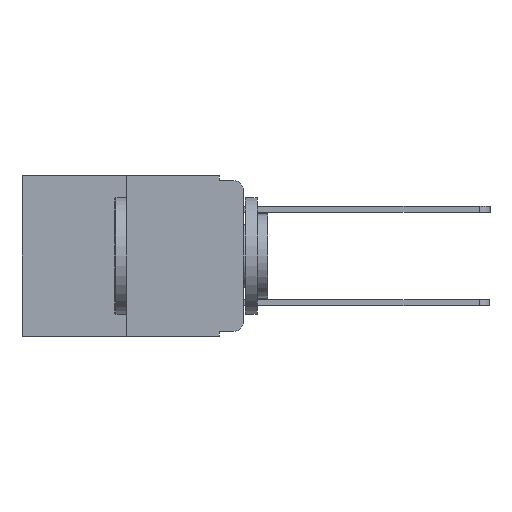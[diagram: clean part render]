
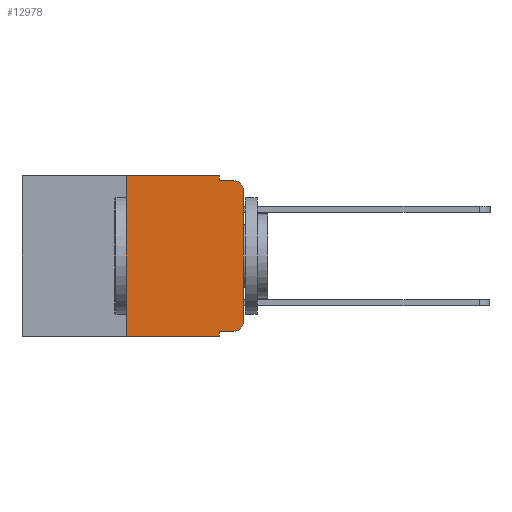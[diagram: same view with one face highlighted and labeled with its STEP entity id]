
A CAD part, left-side view. The second image highlights one B-rep face of the part: STEP entity #12978.
In plain terms, the highlighted planar face has unit normal (-1, 0, 0).
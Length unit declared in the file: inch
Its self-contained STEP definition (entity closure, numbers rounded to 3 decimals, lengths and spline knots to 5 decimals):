
#247 = DIRECTION ( 'NONE',  ( 0., 0., -1. ) ) ;
#1131 = DIRECTION ( 'NONE',  ( 0., 0., 1. ) ) ;
#1620 = CARTESIAN_POINT ( 'NONE',  ( 0., 0.051, 0. ) ) ;
#1825 = DIRECTION ( 'NONE',  ( -1., 0., 0. ) ) ;
#1891 = EDGE_CURVE ( 'NONE', #11463, #6679, #20076, .T. ) ;
#2016 = VERTEX_POINT ( 'NONE', #11448 ) ;
#2154 = ORIENTED_EDGE ( 'NONE', *, *, #18420, .F. ) ;
#2264 = AXIS2_PLACEMENT_3D ( 'NONE', #14364, #10949, #247 ) ;
#2492 = CARTESIAN_POINT ( 'NONE',  ( 0., 0.051, -0.01 ) ) ;
#2641 = CARTESIAN_POINT ( 'NONE',  ( 0., 0., -0.313 ) ) ;
#2963 = CARTESIAN_POINT ( 'NONE',  ( 0., 0.25, 0. ) ) ;
#3008 = DIRECTION ( 'NONE',  ( 0., -1., 0. ) ) ;
#3099 = DIRECTION ( 'NONE',  ( 0., -1., 0. ) ) ;
#3261 = CARTESIAN_POINT ( 'NONE',  ( 0., 0., -0.03 ) ) ;
#3526 = LINE ( 'NONE', #5634, #20583 ) ;
#4496 = ORIENTED_EDGE ( 'NONE', *, *, #16631, .F. ) ;
#4811 = AXIS2_PLACEMENT_3D ( 'NONE', #21503, #11521, #12048 ) ;
#4846 = VECTOR ( 'NONE', #18202, 39.37008 ) ;
#4972 = EDGE_CURVE ( 'NONE', #9702, #18778, #13136, .T. ) ;
#5262 = FACE_OUTER_BOUND ( 'NONE', #18132, .T. ) ;
#5592 = CARTESIAN_POINT ( 'NONE',  ( 0., 0.051, 0. ) ) ;
#5634 = CARTESIAN_POINT ( 'NONE',  ( 0., 0., 0. ) ) ;
#6679 = VERTEX_POINT ( 'NONE', #20469 ) ;
#6851 = EDGE_CURVE ( 'NONE', #20647, #14559, #3526, .T. ) ;
#6977 = LINE ( 'NONE', #1620, #12164 ) ;
#7351 = DIRECTION ( 'NONE',  ( 0., 0., 1. ) ) ;
#7438 = VERTEX_POINT ( 'NONE', #17466 ) ;
#8669 = EDGE_CURVE ( 'NONE', #12293, #20647, #12718, .T. ) ;
#8773 = ORIENTED_EDGE ( 'NONE', *, *, #6851, .T. ) ;
#9199 = CARTESIAN_POINT ( 'NONE',  ( 0., 0.051, -0.01 ) ) ;
#9393 = ORIENTED_EDGE ( 'NONE', *, *, #12486, .T. ) ;
#9610 = EDGE_CURVE ( 'NONE', #14559, #18778, #20460, .T. ) ;
#9702 = VERTEX_POINT ( 'NONE', #2492 ) ;
#10206 = VERTEX_POINT ( 'NONE', #5592 ) ;
#10754 = ORIENTED_EDGE ( 'NONE', *, *, #16348, .F. ) ;
#10949 = DIRECTION ( 'NONE',  ( 1., 0., 0. ) ) ;
#11448 = CARTESIAN_POINT ( 'NONE',  ( 0., 0.051, -0.333 ) ) ;
#11463 = VERTEX_POINT ( 'NONE', #19339 ) ;
#11521 = DIRECTION ( 'NONE',  ( -1., 0., 0. ) ) ;
#11679 = VECTOR ( 'NONE', #1131, 39.37008 ) ;
#12048 = DIRECTION ( 'NONE',  ( 0., 0., -1. ) ) ;
#12164 = VECTOR ( 'NONE', #13946, 39.37008 ) ;
#12293 = VERTEX_POINT ( 'NONE', #16423 ) ;
#12345 = VECTOR ( 'NONE', #3008, 39.37008 ) ;
#12403 = CARTESIAN_POINT ( 'NONE',  ( 0., 0.02, -0.313 ) ) ;
#12486 = EDGE_CURVE ( 'NONE', #2016, #12293, #16590, .T. ) ;
#12650 = EDGE_CURVE ( 'NONE', #7438, #10206, #16335, .T. ) ;
#12718 = CIRCLE ( 'NONE', #15774, 0.02 ) ;
#12727 = DIRECTION ( 'NONE',  ( 0., -1., 0. ) ) ;
#12978 = ADVANCED_FACE ( 'NONE', ( #5262 ), #16028, .F. ) ;
#13136 = LINE ( 'NONE', #9199, #21398 ) ;
#13228 = ORIENTED_EDGE ( 'NONE', *, *, #9610, .T. ) ;
#13432 = ORIENTED_EDGE ( 'NONE', *, *, #12650, .F. ) ;
#13772 = ORIENTED_EDGE ( 'NONE', *, *, #8669, .T. ) ;
#13946 = DIRECTION ( 'NONE',  ( 0., 0., -1. ) ) ;
#13992 = CARTESIAN_POINT ( 'NONE',  ( 0., 0.473, 0. ) ) ;
#14143 = DIRECTION ( 'NONE',  ( 0., 0., -1. ) ) ;
#14364 = CARTESIAN_POINT ( 'NONE',  ( 0., 0.473, 0. ) ) ;
#14559 = VERTEX_POINT ( 'NONE', #3261 ) ;
#15557 = VECTOR ( 'NONE', #3099, 39.37008 ) ;
#15702 = DIRECTION ( 'NONE',  ( 0., -1., 0. ) ) ;
#15704 = VECTOR ( 'NONE', #15702, 39.37008 ) ;
#15774 = AXIS2_PLACEMENT_3D ( 'NONE', #12403, #1825, #14143 ) ;
#15867 = ORIENTED_EDGE ( 'NONE', *, *, #4972, .F. ) ;
#15917 = CARTESIAN_POINT ( 'NONE',  ( 0., 0.473, -0.343 ) ) ;
#16028 = PLANE ( 'NONE',  #2264 ) ;
#16335 = LINE ( 'NONE', #13992, #12345 ) ;
#16348 = EDGE_CURVE ( 'NONE', #2016, #6679, #18509, .T. ) ;
#16423 = CARTESIAN_POINT ( 'NONE',  ( 0., 0.02, -0.333 ) ) ;
#16521 = CARTESIAN_POINT ( 'NONE',  ( 0., 0.051, 0. ) ) ;
#16590 = LINE ( 'NONE', #16919, #15557 ) ;
#16631 = EDGE_CURVE ( 'NONE', #10206, #9702, #6977, .T. ) ;
#16919 = CARTESIAN_POINT ( 'NONE',  ( 0., 0.051, -0.333 ) ) ;
#17466 = CARTESIAN_POINT ( 'NONE',  ( 0., 0.25, 0. ) ) ;
#18132 = EDGE_LOOP ( 'NONE', ( #8773, #13228, #15867, #4496, #13432, #2154, #19456, #10754, #9393, #13772 ) ) ;
#18202 = DIRECTION ( 'NONE',  ( 0., 0., -1. ) ) ;
#18420 = EDGE_CURVE ( 'NONE', #11463, #7438, #21069, .T. ) ;
#18509 = LINE ( 'NONE', #16521, #4846 ) ;
#18778 = VERTEX_POINT ( 'NONE', #20995 ) ;
#19339 = CARTESIAN_POINT ( 'NONE',  ( 0., 0.25, -0.343 ) ) ;
#19456 = ORIENTED_EDGE ( 'NONE', *, *, #1891, .T. ) ;
#20076 = LINE ( 'NONE', #15917, #15704 ) ;
#20460 = CIRCLE ( 'NONE', #4811, 0.02 ) ;
#20469 = CARTESIAN_POINT ( 'NONE',  ( 0., 0.051, -0.343 ) ) ;
#20583 = VECTOR ( 'NONE', #7351, 39.37008 ) ;
#20647 = VERTEX_POINT ( 'NONE', #2641 ) ;
#20995 = CARTESIAN_POINT ( 'NONE',  ( 0., 0.02, -0.01 ) ) ;
#21069 = LINE ( 'NONE', #2963, #11679 ) ;
#21398 = VECTOR ( 'NONE', #12727, 39.37008 ) ;
#21503 = CARTESIAN_POINT ( 'NONE',  ( 0., 0.02, -0.03 ) ) ;
